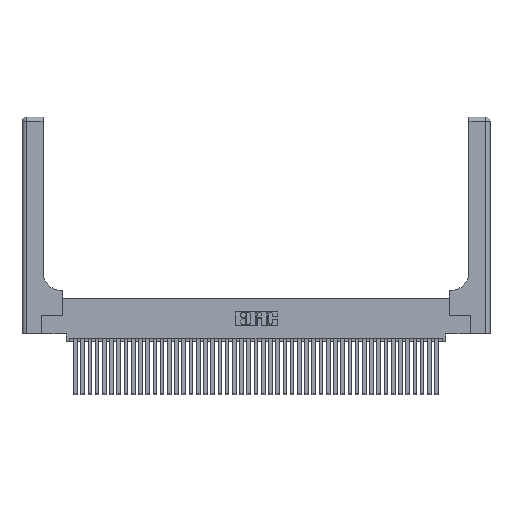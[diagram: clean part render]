
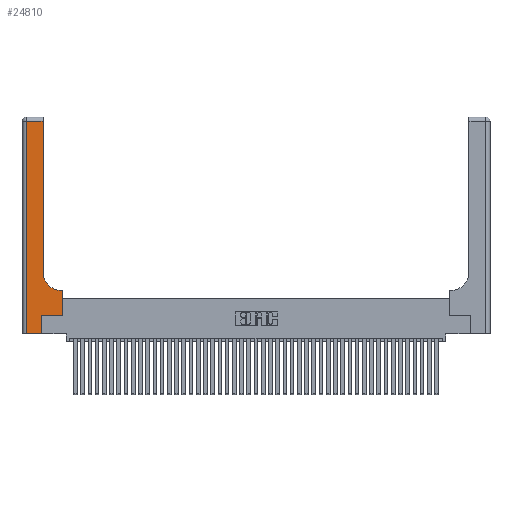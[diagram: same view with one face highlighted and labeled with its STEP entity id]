
A CAD part, top view. The second image highlights one B-rep face of the part: STEP entity #24810.
In plain terms, the highlighted planar face has unit normal (0, 0, 1).
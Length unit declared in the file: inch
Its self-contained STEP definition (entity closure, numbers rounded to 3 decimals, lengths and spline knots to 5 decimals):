
#208 = CARTESIAN_POINT ( 'NONE',  ( 0.2915, 2.94, 0.37 ) ) ;
#649 = CARTESIAN_POINT ( 'NONE',  ( 0.5415, 0.85, 0.37 ) ) ;
#1430 = DIRECTION ( 'NONE',  ( 0., 1., 0. ) ) ;
#2145 = ORIENTED_EDGE ( 'NONE', *, *, #18836, .T. ) ;
#2835 = DIRECTION ( 'NONE',  ( 1., 0., 0. ) ) ;
#3696 = AXIS2_PLACEMENT_3D ( 'NONE', #649, #41176, #10886 ) ;
#4697 = CARTESIAN_POINT ( 'NONE',  ( 0., 2.94, 0.37 ) ) ;
#5239 = CARTESIAN_POINT ( 'NONE',  ( 0.06, 3., 0.37 ) ) ;
#6185 = CARTESIAN_POINT ( 'NONE',  ( 0.5585, 0.25, 0.37 ) ) ;
#7488 = ORIENTED_EDGE ( 'NONE', *, *, #15988, .T. ) ;
#7555 = LINE ( 'NONE', #39278, #10761 ) ;
#7829 = VERTEX_POINT ( 'NONE', #17788 ) ;
#7916 = CARTESIAN_POINT ( 'NONE',  ( 0.06, 2.94, 0.37 ) ) ;
#8585 = EDGE_CURVE ( 'NONE', #13323, #33042, #15644, .T. ) ;
#9724 = VERTEX_POINT ( 'NONE', #22062 ) ;
#10761 = VECTOR ( 'NONE', #1430, 39.37008 ) ;
#10886 = DIRECTION ( 'NONE',  ( 1., 0., 0. ) ) ;
#13323 = VERTEX_POINT ( 'NONE', #40960 ) ;
#13682 = VERTEX_POINT ( 'NONE', #7916 ) ;
#14538 = VECTOR ( 'NONE', #33193, 39.37008 ) ;
#15048 = VERTEX_POINT ( 'NONE', #35604 ) ;
#15644 = CIRCLE ( 'NONE', #3696, 0.25 ) ;
#15677 = EDGE_CURVE ( 'NONE', #15048, #9724, #41620, .T. ) ;
#15988 = EDGE_CURVE ( 'NONE', #33042, #29967, #7555, .T. ) ;
#16027 = LINE ( 'NONE', #6185, #40432 ) ;
#16436 = VERTEX_POINT ( 'NONE', #27586 ) ;
#17697 = LINE ( 'NONE', #41002, #42672 ) ;
#17788 = CARTESIAN_POINT ( 'NONE',  ( 0.5585, 0.6, 0.37 ) ) ;
#18836 = EDGE_CURVE ( 'NONE', #16436, #15048, #23527, .T. ) ;
#19668 = ORIENTED_EDGE ( 'NONE', *, *, #15677, .T. ) ;
#20683 = ORIENTED_EDGE ( 'NONE', *, *, #8585, .T. ) ;
#21050 = CARTESIAN_POINT ( 'NONE',  ( 0., 3., 0.37 ) ) ;
#21206 = DIRECTION ( 'NONE',  ( 0., 0., -1. ) ) ;
#22062 = CARTESIAN_POINT ( 'NONE',  ( 0.269, 0.25, 0.37 ) ) ;
#22654 = LINE ( 'NONE', #5239, #40102 ) ;
#23149 = VECTOR ( 'NONE', #39033, 39.37008 ) ;
#23527 = LINE ( 'NONE', #43540, #28290 ) ;
#24397 = DIRECTION ( 'NONE',  ( 1., 0., 0. ) ) ;
#24611 = DIRECTION ( 'NONE',  ( -1., 0., 0. ) ) ;
#24810 = ADVANCED_FACE ( 'NONE', ( #28144 ), #41516, .F. ) ;
#25861 = AXIS2_PLACEMENT_3D ( 'NONE', #21050, #21206, #24611 ) ;
#27109 = CARTESIAN_POINT ( 'NONE',  ( 0.5585, 0.25, 0.37 ) ) ;
#27260 = ORIENTED_EDGE ( 'NONE', *, *, #28877, .T. ) ;
#27586 = CARTESIAN_POINT ( 'NONE',  ( 0.06, 0., 0.37 ) ) ;
#27705 = EDGE_LOOP ( 'NONE', ( #7488, #28491, #36055, #2145, #19668, #27260, #33740, #41522, #20683 ) ) ;
#28022 = EDGE_CURVE ( 'NONE', #29967, #13682, #43310, .T. ) ;
#28144 = FACE_OUTER_BOUND ( 'NONE', #27705, .T. ) ;
#28290 = VECTOR ( 'NONE', #2835, 39.37008 ) ;
#28491 = ORIENTED_EDGE ( 'NONE', *, *, #28022, .T. ) ;
#28877 = EDGE_CURVE ( 'NONE', #9724, #37623, #17697, .T. ) ;
#29044 = DIRECTION ( 'NONE',  ( 0., -1., 0. ) ) ;
#29076 = CARTESIAN_POINT ( 'NONE',  ( 0.269, 0., 0.37 ) ) ;
#29825 = CARTESIAN_POINT ( 'NONE',  ( 0.2915, 0.85, 0.37 ) ) ;
#29930 = VECTOR ( 'NONE', #30951, 39.37008 ) ;
#29967 = VERTEX_POINT ( 'NONE', #208 ) ;
#30951 = DIRECTION ( 'NONE',  ( -1., 0., 0. ) ) ;
#31352 = EDGE_CURVE ( 'NONE', #7829, #13323, #40006, .T. ) ;
#32424 = EDGE_CURVE ( 'NONE', #37623, #7829, #16027, .T. ) ;
#33042 = VERTEX_POINT ( 'NONE', #29825 ) ;
#33193 = DIRECTION ( 'NONE',  ( 0., 1., 0. ) ) ;
#33740 = ORIENTED_EDGE ( 'NONE', *, *, #32424, .T. ) ;
#35604 = CARTESIAN_POINT ( 'NONE',  ( 0.269, 0., 0.37 ) ) ;
#36055 = ORIENTED_EDGE ( 'NONE', *, *, #42047, .T. ) ;
#37623 = VERTEX_POINT ( 'NONE', #27109 ) ;
#37930 = CARTESIAN_POINT ( 'NONE',  ( 0.2915, 0.6, 0.37 ) ) ;
#39033 = DIRECTION ( 'NONE',  ( -1., 0., 0. ) ) ;
#39278 = CARTESIAN_POINT ( 'NONE',  ( 0.2915, 3., 0.37 ) ) ;
#40006 = LINE ( 'NONE', #37930, #29930 ) ;
#40102 = VECTOR ( 'NONE', #29044, 39.37008 ) ;
#40364 = DIRECTION ( 'NONE',  ( 0., 1., 0. ) ) ;
#40432 = VECTOR ( 'NONE', #40364, 39.37008 ) ;
#40960 = CARTESIAN_POINT ( 'NONE',  ( 0.5415, 0.6, 0.37 ) ) ;
#41002 = CARTESIAN_POINT ( 'NONE',  ( 0.269, 0.25, 0.37 ) ) ;
#41176 = DIRECTION ( 'NONE',  ( 0., 0., -1. ) ) ;
#41516 = PLANE ( 'NONE',  #25861 ) ;
#41522 = ORIENTED_EDGE ( 'NONE', *, *, #31352, .T. ) ;
#41620 = LINE ( 'NONE', #29076, #14538 ) ;
#42047 = EDGE_CURVE ( 'NONE', #13682, #16436, #22654, .T. ) ;
#42672 = VECTOR ( 'NONE', #24397, 39.37008 ) ;
#43310 = LINE ( 'NONE', #4697, #23149 ) ;
#43540 = CARTESIAN_POINT ( 'NONE',  ( 0., 0., 0.37 ) ) ;
